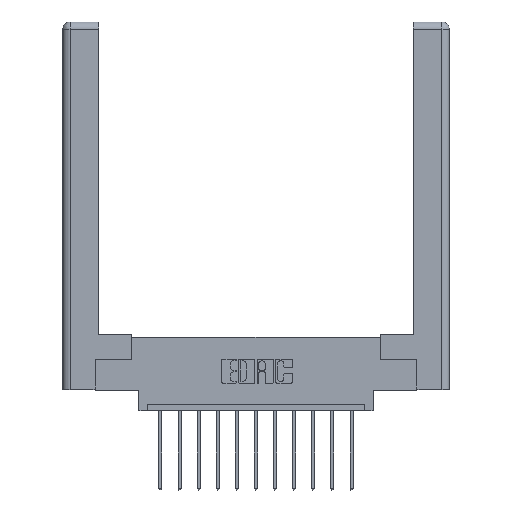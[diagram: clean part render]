
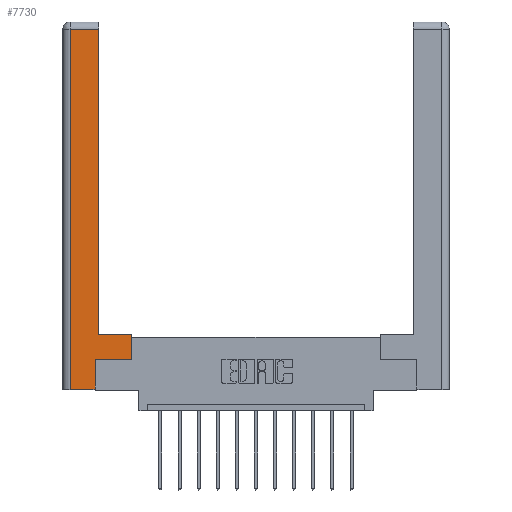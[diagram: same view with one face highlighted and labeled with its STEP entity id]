
A CAD part, top view. The second image highlights one B-rep face of the part: STEP entity #7730.
In plain terms, the highlighted planar face has unit normal (0, 0, 1).
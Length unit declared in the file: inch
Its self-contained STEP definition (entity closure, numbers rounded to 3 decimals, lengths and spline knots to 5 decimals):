
#204 = LINE ( 'NONE', #2981, #11998 ) ;
#448 = LINE ( 'NONE', #12557, #14749 ) ;
#458 = VERTEX_POINT ( 'NONE', #4937 ) ;
#968 = DIRECTION ( 'NONE',  ( -1., 0., 0. ) ) ;
#1439 = VECTOR ( 'NONE', #7130, 39.37008 ) ;
#1446 = VERTEX_POINT ( 'NONE', #4547 ) ;
#1505 = VERTEX_POINT ( 'NONE', #12871 ) ;
#1833 = LINE ( 'NONE', #9183, #3084 ) ;
#1933 = CARTESIAN_POINT ( 'NONE',  ( 0.295, 0.45, 0. ) ) ;
#1939 = VECTOR ( 'NONE', #13282, 39.37008 ) ;
#2039 = ORIENTED_EDGE ( 'NONE', *, *, #9131, .T. ) ;
#2135 = PLANE ( 'NONE',  #3803 ) ;
#2655 = EDGE_LOOP ( 'NONE', ( #12342, #8170, #2039, #4291, #13937, #13568, #4243, #14682 ) ) ;
#2930 = VECTOR ( 'NONE', #9789, 39.37008 ) ;
#2981 = CARTESIAN_POINT ( 'NONE',  ( 0.295, 3., 0. ) ) ;
#3020 = LINE ( 'NONE', #6252, #1939 ) ;
#3084 = VECTOR ( 'NONE', #6900, 39.37008 ) ;
#3627 = CARTESIAN_POINT ( 'NONE',  ( 0.565, 0.45, 0. ) ) ;
#3803 = AXIS2_PLACEMENT_3D ( 'NONE', #14956, #4523, #4572 ) ;
#4206 = DIRECTION ( 'NONE',  ( 1., 0., 0. ) ) ;
#4243 = ORIENTED_EDGE ( 'NONE', *, *, #5996, .T. ) ;
#4291 = ORIENTED_EDGE ( 'NONE', *, *, #4677, .T. ) ;
#4449 = VECTOR ( 'NONE', #6422, 39.37008 ) ;
#4523 = DIRECTION ( 'NONE',  ( 0., 0., -1. ) ) ;
#4547 = CARTESIAN_POINT ( 'NONE',  ( 0.565, 0.245, 0. ) ) ;
#4572 = DIRECTION ( 'NONE',  ( -1., 0., 0. ) ) ;
#4677 = EDGE_CURVE ( 'NONE', #11676, #458, #5995, .T. ) ;
#4937 = CARTESIAN_POINT ( 'NONE',  ( 0.265, 0., 0. ) ) ;
#5995 = LINE ( 'NONE', #8579, #2930 ) ;
#5996 = EDGE_CURVE ( 'NONE', #1446, #13634, #6716, .T. ) ;
#6252 = CARTESIAN_POINT ( 'NONE',  ( 0.265, 0.245, 0. ) ) ;
#6422 = DIRECTION ( 'NONE',  ( -1., 0., 0. ) ) ;
#6716 = LINE ( 'NONE', #3627, #1439 ) ;
#6900 = DIRECTION ( 'NONE',  ( 0., -1., 0. ) ) ;
#7130 = DIRECTION ( 'NONE',  ( 0., 1., 0. ) ) ;
#7322 = VECTOR ( 'NONE', #4206, 39.37008 ) ;
#7340 = LINE ( 'NONE', #9837, #4449 ) ;
#7730 = ADVANCED_FACE ( 'NONE', ( #8667 ), #2135, .F. ) ;
#8159 = EDGE_CURVE ( 'NONE', #10257, #1505, #204, .T. ) ;
#8170 = ORIENTED_EDGE ( 'NONE', *, *, #12562, .T. ) ;
#8579 = CARTESIAN_POINT ( 'NONE',  ( 0.265, 0., 0. ) ) ;
#8667 = FACE_OUTER_BOUND ( 'NONE', #2655, .T. ) ;
#9131 = EDGE_CURVE ( 'NONE', #14343, #11676, #1833, .T. ) ;
#9183 = CARTESIAN_POINT ( 'NONE',  ( 0.0615, 0., 0. ) ) ;
#9789 = DIRECTION ( 'NONE',  ( 1., 0., 0. ) ) ;
#9837 = CARTESIAN_POINT ( 'NONE',  ( 0.0615, 2.94, 0. ) ) ;
#10257 = VERTEX_POINT ( 'NONE', #1933 ) ;
#11033 = DIRECTION ( 'NONE',  ( 0., 1., 0. ) ) ;
#11207 = CARTESIAN_POINT ( 'NONE',  ( 0.565, 0.45, 0. ) ) ;
#11458 = CARTESIAN_POINT ( 'NONE',  ( 0.0615, 2.94, 0. ) ) ;
#11676 = VERTEX_POINT ( 'NONE', #14741 ) ;
#11998 = VECTOR ( 'NONE', #11033, 39.37008 ) ;
#12025 = EDGE_CURVE ( 'NONE', #458, #12545, #3020, .T. ) ;
#12342 = ORIENTED_EDGE ( 'NONE', *, *, #8159, .T. ) ;
#12545 = VERTEX_POINT ( 'NONE', #14350 ) ;
#12557 = CARTESIAN_POINT ( 'NONE',  ( 0.295, 0.45, 0. ) ) ;
#12562 = EDGE_CURVE ( 'NONE', #1505, #14343, #7340, .T. ) ;
#12871 = CARTESIAN_POINT ( 'NONE',  ( 0.295, 2.94, 0. ) ) ;
#13186 = EDGE_CURVE ( 'NONE', #12545, #1446, #14193, .T. ) ;
#13282 = DIRECTION ( 'NONE',  ( 0., 1., 0. ) ) ;
#13401 = CARTESIAN_POINT ( 'NONE',  ( 0.565, 0.245, 0. ) ) ;
#13568 = ORIENTED_EDGE ( 'NONE', *, *, #13186, .T. ) ;
#13634 = VERTEX_POINT ( 'NONE', #11207 ) ;
#13937 = ORIENTED_EDGE ( 'NONE', *, *, #12025, .T. ) ;
#14193 = LINE ( 'NONE', #13401, #7322 ) ;
#14305 = EDGE_CURVE ( 'NONE', #13634, #10257, #448, .T. ) ;
#14343 = VERTEX_POINT ( 'NONE', #11458 ) ;
#14350 = CARTESIAN_POINT ( 'NONE',  ( 0.265, 0.245, 0. ) ) ;
#14682 = ORIENTED_EDGE ( 'NONE', *, *, #14305, .T. ) ;
#14741 = CARTESIAN_POINT ( 'NONE',  ( 0.0615, 0., 0. ) ) ;
#14749 = VECTOR ( 'NONE', #968, 39.37008 ) ;
#14956 = CARTESIAN_POINT ( 'NONE',  ( 0., 0., 0. ) ) ;
